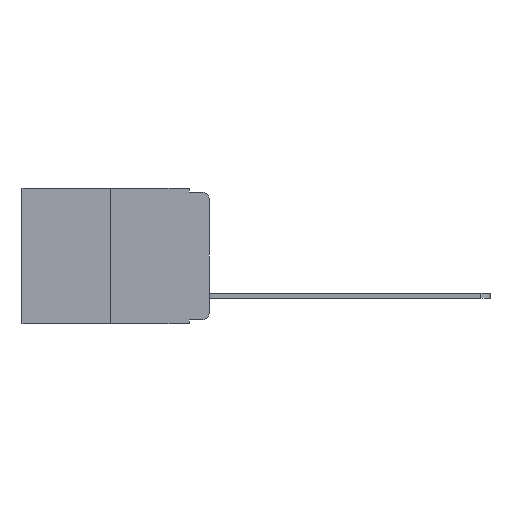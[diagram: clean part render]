
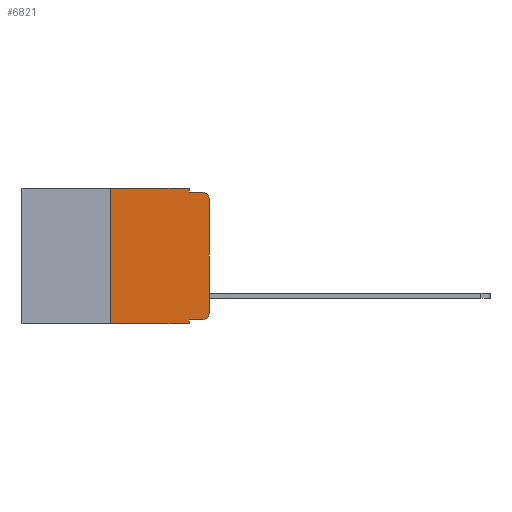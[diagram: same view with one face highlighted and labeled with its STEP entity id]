
A CAD part, left-side view. The second image highlights one B-rep face of the part: STEP entity #6821.
In plain terms, the highlighted planar face has unit normal (-1, 0, 0).
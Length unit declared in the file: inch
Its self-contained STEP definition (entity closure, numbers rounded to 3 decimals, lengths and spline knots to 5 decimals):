
#24 = EDGE_CURVE ( 'NONE', #2438, #3193, #5631, .T. ) ;
#220 = DIRECTION ( 'NONE',  ( 0., 0., 1. ) ) ;
#447 = DIRECTION ( 'NONE',  ( 0., -1., 0. ) ) ;
#547 = EDGE_CURVE ( 'NONE', #6873, #2271, #3765, .T. ) ;
#612 = CARTESIAN_POINT ( 'NONE',  ( 0., 0.051, -0.333 ) ) ;
#756 = EDGE_CURVE ( 'NONE', #2133, #1569, #4571, .T. ) ;
#1043 = ORIENTED_EDGE ( 'NONE', *, *, #3944, .T. ) ;
#1088 = VERTEX_POINT ( 'NONE', #7211 ) ;
#1093 = VERTEX_POINT ( 'NONE', #8723 ) ;
#1112 = ORIENTED_EDGE ( 'NONE', *, *, #4061, .F. ) ;
#1182 = ORIENTED_EDGE ( 'NONE', *, *, #3960, .T. ) ;
#1183 = CARTESIAN_POINT ( 'NONE',  ( 0., 0.02, -0.313 ) ) ;
#1238 = ORIENTED_EDGE ( 'NONE', *, *, #24, .F. ) ;
#1282 = ORIENTED_EDGE ( 'NONE', *, *, #5619, .F. ) ;
#1285 = DIRECTION ( 'NONE',  ( 0., 0., -1. ) ) ;
#1294 = ORIENTED_EDGE ( 'NONE', *, *, #547, .F. ) ;
#1362 = ORIENTED_EDGE ( 'NONE', *, *, #756, .F. ) ;
#1413 = VECTOR ( 'NONE', #7133, 39.37008 ) ;
#1422 = ORIENTED_EDGE ( 'NONE', *, *, #6793, .T. ) ;
#1437 = ORIENTED_EDGE ( 'NONE', *, *, #6917, .T. ) ;
#1569 = VERTEX_POINT ( 'NONE', #3429 ) ;
#1640 = DIRECTION ( 'NONE',  ( 0., 0., -1. ) ) ;
#1864 = EDGE_LOOP ( 'NONE', ( #1043, #1182, #1112, #1238, #1282, #1294, #2161, #1362, #1437, #1422 ) ) ;
#1951 = CIRCLE ( 'NONE', #6625, 0.02 ) ;
#1954 = EDGE_CURVE ( 'NONE', #6873, #1569, #3478, .T. ) ;
#2133 = VERTEX_POINT ( 'NONE', #7525 ) ;
#2161 = ORIENTED_EDGE ( 'NONE', *, *, #1954, .T. ) ;
#2271 = VERTEX_POINT ( 'NONE', #2560 ) ;
#2307 = CARTESIAN_POINT ( 'NONE',  ( 0., 0.25, -0.343 ) ) ;
#2366 = CARTESIAN_POINT ( 'NONE',  ( 0., 0.473, 0. ) ) ;
#2438 = VERTEX_POINT ( 'NONE', #7926 ) ;
#2472 = VECTOR ( 'NONE', #1640, 39.37008 ) ;
#2560 = CARTESIAN_POINT ( 'NONE',  ( 0., 0.25, 0. ) ) ;
#2570 = PLANE ( 'NONE',  #5737 ) ;
#2578 = DIRECTION ( 'NONE',  ( -1., 0., 0. ) ) ;
#2582 = LINE ( 'NONE', #612, #6330 ) ;
#2615 = DIRECTION ( 'NONE',  ( 0., 0., -1. ) ) ;
#2675 = DIRECTION ( 'NONE',  ( 1., 0., 0. ) ) ;
#2780 = CARTESIAN_POINT ( 'NONE',  ( 0., 0., -0.03 ) ) ;
#2869 = CARTESIAN_POINT ( 'NONE',  ( 0., 0.02, -0.333 ) ) ;
#3006 = LINE ( 'NONE', #3203, #6663 ) ;
#3060 = LINE ( 'NONE', #6551, #6716 ) ;
#3193 = VERTEX_POINT ( 'NONE', #5763 ) ;
#3203 = CARTESIAN_POINT ( 'NONE',  ( 0., 0.051, -0.01 ) ) ;
#3429 = CARTESIAN_POINT ( 'NONE',  ( 0., 0.051, -0.343 ) ) ;
#3478 = LINE ( 'NONE', #6146, #1413 ) ;
#3660 = DIRECTION ( 'NONE',  ( 0., 0., -1. ) ) ;
#3765 = LINE ( 'NONE', #4069, #5610 ) ;
#3944 = EDGE_CURVE ( 'NONE', #1088, #8725, #6180, .T. ) ;
#3960 = EDGE_CURVE ( 'NONE', #8725, #1093, #1951, .T. ) ;
#4061 = EDGE_CURVE ( 'NONE', #3193, #1093, #3006, .T. ) ;
#4066 = DIRECTION ( 'NONE',  ( 0., 0., 1. ) ) ;
#4069 = CARTESIAN_POINT ( 'NONE',  ( 0., 0.25, 0. ) ) ;
#4436 = DIRECTION ( 'NONE',  ( -1., 0., 0. ) ) ;
#4466 = CARTESIAN_POINT ( 'NONE',  ( 0., 0., 0. ) ) ;
#4496 = VECTOR ( 'NONE', #220, 39.37008 ) ;
#4571 = LINE ( 'NONE', #5627, #2472 ) ;
#5589 = DIRECTION ( 'NONE',  ( 0., -1., 0. ) ) ;
#5610 = VECTOR ( 'NONE', #4066, 39.37008 ) ;
#5619 = EDGE_CURVE ( 'NONE', #2271, #2438, #3060, .T. ) ;
#5627 = CARTESIAN_POINT ( 'NONE',  ( 0., 0.051, 0. ) ) ;
#5631 = LINE ( 'NONE', #7469, #8671 ) ;
#5737 = AXIS2_PLACEMENT_3D ( 'NONE', #2366, #2675, #2615 ) ;
#5763 = CARTESIAN_POINT ( 'NONE',  ( 0., 0.051, -0.01 ) ) ;
#5772 = AXIS2_PLACEMENT_3D ( 'NONE', #1183, #2578, #1285 ) ;
#6146 = CARTESIAN_POINT ( 'NONE',  ( 0., 0.473, -0.343 ) ) ;
#6180 = LINE ( 'NONE', #4466, #4496 ) ;
#6330 = VECTOR ( 'NONE', #447, 39.37008 ) ;
#6444 = DIRECTION ( 'NONE',  ( 0., -1., 0. ) ) ;
#6515 = VERTEX_POINT ( 'NONE', #2869 ) ;
#6551 = CARTESIAN_POINT ( 'NONE',  ( 0., 0.473, 0. ) ) ;
#6561 = CARTESIAN_POINT ( 'NONE',  ( 0., 0.02, -0.03 ) ) ;
#6625 = AXIS2_PLACEMENT_3D ( 'NONE', #6561, #4436, #3660 ) ;
#6658 = DIRECTION ( 'NONE',  ( 0., 0., -1. ) ) ;
#6663 = VECTOR ( 'NONE', #5589, 39.37008 ) ;
#6708 = CIRCLE ( 'NONE', #5772, 0.02 ) ;
#6716 = VECTOR ( 'NONE', #6444, 39.37008 ) ;
#6793 = EDGE_CURVE ( 'NONE', #6515, #1088, #6708, .T. ) ;
#6821 = ADVANCED_FACE ( 'NONE', ( #8286 ), #2570, .F. ) ;
#6873 = VERTEX_POINT ( 'NONE', #2307 ) ;
#6917 = EDGE_CURVE ( 'NONE', #2133, #6515, #2582, .T. ) ;
#7133 = DIRECTION ( 'NONE',  ( 0., -1., 0. ) ) ;
#7211 = CARTESIAN_POINT ( 'NONE',  ( 0., 0., -0.313 ) ) ;
#7469 = CARTESIAN_POINT ( 'NONE',  ( 0., 0.051, 0. ) ) ;
#7525 = CARTESIAN_POINT ( 'NONE',  ( 0., 0.051, -0.333 ) ) ;
#7926 = CARTESIAN_POINT ( 'NONE',  ( 0., 0.051, 0. ) ) ;
#8286 = FACE_OUTER_BOUND ( 'NONE', #1864, .T. ) ;
#8671 = VECTOR ( 'NONE', #6658, 39.37008 ) ;
#8723 = CARTESIAN_POINT ( 'NONE',  ( 0., 0.02, -0.01 ) ) ;
#8725 = VERTEX_POINT ( 'NONE', #2780 ) ;
